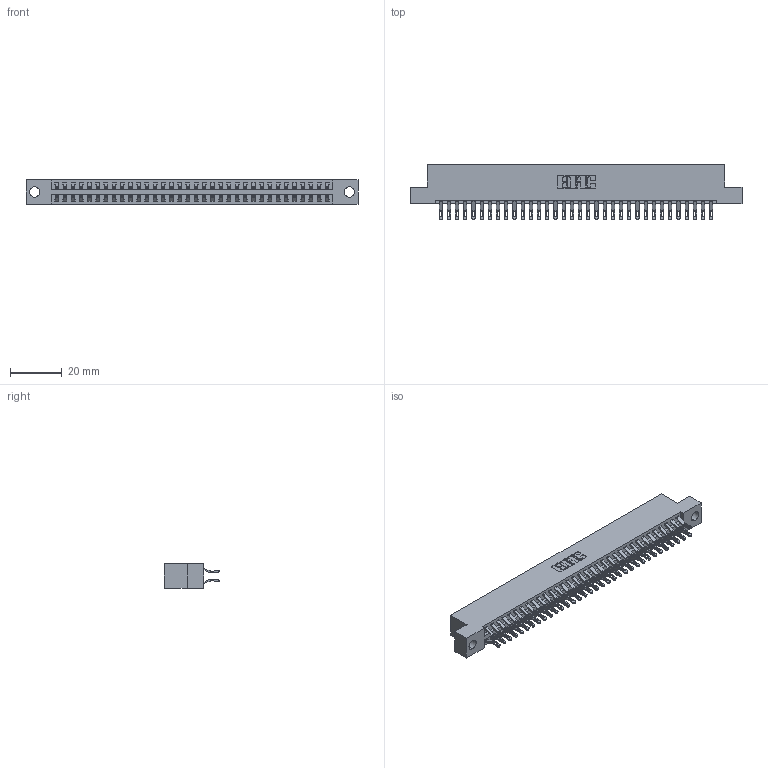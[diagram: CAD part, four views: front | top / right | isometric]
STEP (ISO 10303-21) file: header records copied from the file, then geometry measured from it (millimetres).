
FILE_DESCRIPTION (( 'STEP AP203' ), '1' );
FILE_NAME ('346-068-555-204.STEP', '2022-05-24T19:38:35', ( '' ), ( '' ), 'SwSTEP 2.0', 'SolidWorks 2020', '' );
FILE_SCHEMA (( 'CONFIG_CONTROL_DESIGN' ));
Length unit declared in the file: inch
Products named in the file (3): 346-068-555-204; 345-292-001_555 Tail; 346 Part_Flush Mounting Lugs - 0.156 Dia-TH
Assembly tree (69 placements, depth 2):
  346-068-555-204
    346 Part_Flush Mounting Lugs - 0.156 Dia-TH
    345-292-001_555 Tail  x68
Bounding box: 128.52 x 21.46 x 9.4 mm (x, y, z)
Volume: 12561.8 mm3; surface area: 17692.3 mm2
Topology: 69 solids, 69 shells, 4080 faces, 12809 edges, 8538 vertices
Faces by surface type: plane 2334, cylinder 1746
Entity records: 24011 total; most frequent: CARTESIAN_POINT 4008, ORIENTED_EDGE 3910, DIRECTION 3551, EDGE_CURVE 1955, VECTOR 1667, LINE 1667, VERTEX_POINT 1302, AXIS2_PLACEMENT_3D 942
